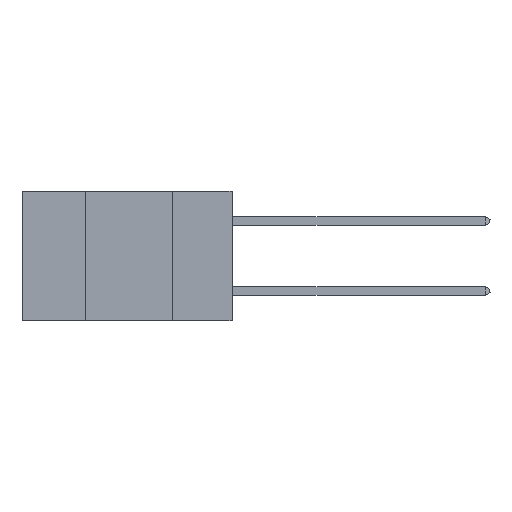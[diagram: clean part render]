
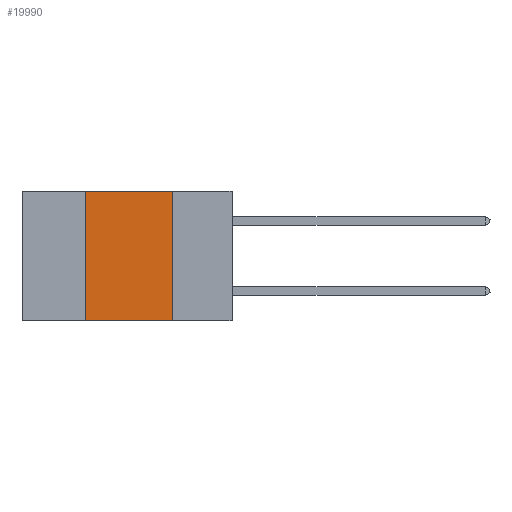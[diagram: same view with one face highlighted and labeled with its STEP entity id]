
A CAD part, left-side view. The second image highlights one B-rep face of the part: STEP entity #19990.
In plain terms, the highlighted planar face has unit normal (-1, 0, 0).
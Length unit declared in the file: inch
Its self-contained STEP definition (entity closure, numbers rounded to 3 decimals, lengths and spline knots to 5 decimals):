
#3949 = CARTESIAN_POINT ( 'NONE',  ( 0., 0.17, 0. ) ) ;
#4676 = CARTESIAN_POINT ( 'NONE',  ( 0., 0.42, 0. ) ) ;
#4972 = CARTESIAN_POINT ( 'NONE',  ( 0., 0.42, 0. ) ) ;
#7356 = ORIENTED_EDGE ( 'NONE', *, *, #11453, .F. ) ;
#8498 = VERTEX_POINT ( 'NONE', #3949 ) ;
#8578 = VECTOR ( 'NONE', #21922, 39.37008 ) ;
#8742 = DIRECTION ( 'NONE',  ( 0., -1., 0. ) ) ;
#9899 = VERTEX_POINT ( 'NONE', #13163 ) ;
#10807 = AXIS2_PLACEMENT_3D ( 'NONE', #27787, #30452, #19983 ) ;
#11453 = EDGE_CURVE ( 'NONE', #24704, #8498, #29038, .T. ) ;
#11570 = VECTOR ( 'NONE', #12318, 39.37008 ) ;
#12318 = DIRECTION ( 'NONE',  ( 0., -1., 0. ) ) ;
#13163 = CARTESIAN_POINT ( 'NONE',  ( 0., 0.42, -0.37 ) ) ;
#16358 = ORIENTED_EDGE ( 'NONE', *, *, #29033, .F. ) ;
#16366 = LINE ( 'NONE', #21825, #33006 ) ;
#17162 = PLANE ( 'NONE',  #10807 ) ;
#17587 = ORIENTED_EDGE ( 'NONE', *, *, #31720, .T. ) ;
#19983 = DIRECTION ( 'NONE',  ( 0., 0., -1. ) ) ;
#19990 = ADVANCED_FACE ( 'NONE', ( #24187 ), #17162, .F. ) ;
#20053 = VECTOR ( 'NONE', #28572, 39.37008 ) ;
#20215 = CARTESIAN_POINT ( 'NONE',  ( 0., 0.6, 0. ) ) ;
#21825 = CARTESIAN_POINT ( 'NONE',  ( 0., 0.6, -0.37 ) ) ;
#21922 = DIRECTION ( 'NONE',  ( 0., 0., -1. ) ) ;
#24187 = FACE_OUTER_BOUND ( 'NONE', #31326, .T. ) ;
#24704 = VERTEX_POINT ( 'NONE', #4676 ) ;
#25291 = CARTESIAN_POINT ( 'NONE',  ( 0., 0.17, -0.37 ) ) ;
#25311 = EDGE_CURVE ( 'NONE', #9899, #24704, #32095, .T. ) ;
#26964 = CARTESIAN_POINT ( 'NONE',  ( 0., 0.17, 0. ) ) ;
#27292 = LINE ( 'NONE', #26964, #8578 ) ;
#27787 = CARTESIAN_POINT ( 'NONE',  ( 0., 0.6, 0. ) ) ;
#28572 = DIRECTION ( 'NONE',  ( 0., 0., 1. ) ) ;
#29033 = EDGE_CURVE ( 'NONE', #8498, #30776, #27292, .T. ) ;
#29038 = LINE ( 'NONE', #20215, #11570 ) ;
#29791 = ORIENTED_EDGE ( 'NONE', *, *, #25311, .F. ) ;
#30452 = DIRECTION ( 'NONE',  ( 1., 0., 0. ) ) ;
#30776 = VERTEX_POINT ( 'NONE', #25291 ) ;
#31326 = EDGE_LOOP ( 'NONE', ( #16358, #7356, #29791, #17587 ) ) ;
#31720 = EDGE_CURVE ( 'NONE', #9899, #30776, #16366, .T. ) ;
#32095 = LINE ( 'NONE', #4972, #20053 ) ;
#33006 = VECTOR ( 'NONE', #8742, 39.37008 ) ;
